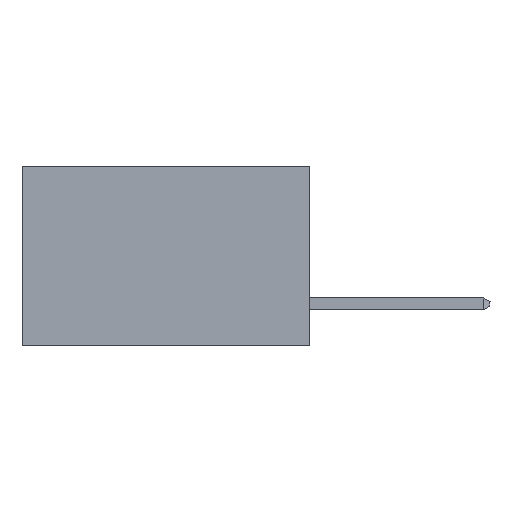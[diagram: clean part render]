
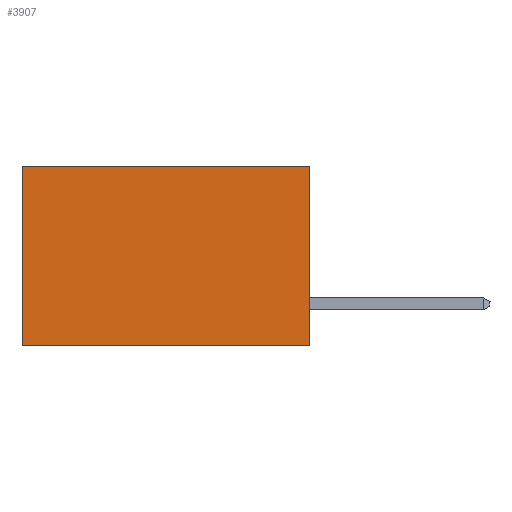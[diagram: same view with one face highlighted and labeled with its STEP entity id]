
A CAD part, left-side view. The second image highlights one B-rep face of the part: STEP entity #3907.
In plain terms, the highlighted planar face has unit normal (-1, 0, 0).
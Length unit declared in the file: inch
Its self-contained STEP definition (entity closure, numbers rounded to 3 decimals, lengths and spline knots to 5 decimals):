
#85 = CARTESIAN_POINT ( 'NONE',  ( 0.2875, 0.6, 0. ) ) ;
#203 = CARTESIAN_POINT ( 'NONE',  ( 0.2875, 0.6, -0.375 ) ) ;
#233 = LINE ( 'NONE', #1373, #1088 ) ;
#300 = PLANE ( 'NONE',  #6357 ) ;
#320 = EDGE_CURVE ( 'NONE', #4967, #7053, #6624, .T. ) ;
#818 = FACE_OUTER_BOUND ( 'NONE', #5565, .T. ) ;
#913 = DIRECTION ( 'NONE',  ( 0., 0., -1. ) ) ;
#947 = CARTESIAN_POINT ( 'NONE',  ( 0.2875, 0., -0.375 ) ) ;
#1079 = VERTEX_POINT ( 'NONE', #203 ) ;
#1088 = VECTOR ( 'NONE', #6983, 39.37008 ) ;
#1301 = ORIENTED_EDGE ( 'NONE', *, *, #5003, .T. ) ;
#1373 = CARTESIAN_POINT ( 'NONE',  ( 0.2875, 0., 0. ) ) ;
#1477 = DIRECTION ( 'NONE',  ( 0., 1., 0. ) ) ;
#2077 = DIRECTION ( 'NONE',  ( 0., 0., -1. ) ) ;
#2804 = VECTOR ( 'NONE', #2077, 39.37008 ) ;
#3428 = CARTESIAN_POINT ( 'NONE',  ( 0.2875, 0., -0.375 ) ) ;
#3846 = VECTOR ( 'NONE', #1477, 39.37008 ) ;
#3907 = ADVANCED_FACE ( 'NONE', ( #818 ), #300, .F. ) ;
#4035 = EDGE_CURVE ( 'NONE', #7406, #1079, #6208, .T. ) ;
#4040 = CARTESIAN_POINT ( 'NONE',  ( 0.2875, 0., -0.375 ) ) ;
#4483 = CARTESIAN_POINT ( 'NONE',  ( 0.2875, 0., 0. ) ) ;
#4639 = LINE ( 'NONE', #4040, #3846 ) ;
#4698 = DIRECTION ( 'NONE',  ( 1., 0., 0. ) ) ;
#4967 = VERTEX_POINT ( 'NONE', #4483 ) ;
#5003 = EDGE_CURVE ( 'NONE', #4967, #7406, #233, .T. ) ;
#5493 = DIRECTION ( 'NONE',  ( 0., 0., -1. ) ) ;
#5565 = EDGE_LOOP ( 'NONE', ( #6094, #7337, #6653, #1301 ) ) ;
#6040 = CARTESIAN_POINT ( 'NONE',  ( 0.2875, 0., -0.375 ) ) ;
#6094 = ORIENTED_EDGE ( 'NONE', *, *, #4035, .T. ) ;
#6208 = LINE ( 'NONE', #7893, #8058 ) ;
#6248 = EDGE_CURVE ( 'NONE', #7053, #1079, #4639, .T. ) ;
#6357 = AXIS2_PLACEMENT_3D ( 'NONE', #947, #4698, #913 ) ;
#6624 = LINE ( 'NONE', #3428, #2804 ) ;
#6653 = ORIENTED_EDGE ( 'NONE', *, *, #320, .F. ) ;
#6983 = DIRECTION ( 'NONE',  ( 0., 1., 0. ) ) ;
#7053 = VERTEX_POINT ( 'NONE', #6040 ) ;
#7337 = ORIENTED_EDGE ( 'NONE', *, *, #6248, .F. ) ;
#7406 = VERTEX_POINT ( 'NONE', #85 ) ;
#7893 = CARTESIAN_POINT ( 'NONE',  ( 0.2875, 0.6, -0.375 ) ) ;
#8058 = VECTOR ( 'NONE', #5493, 39.37008 ) ;
